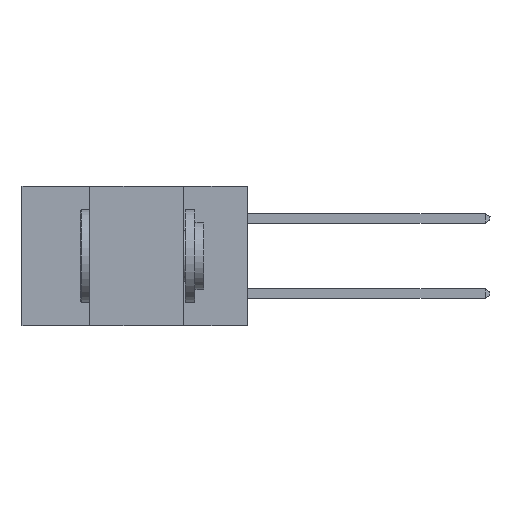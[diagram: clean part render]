
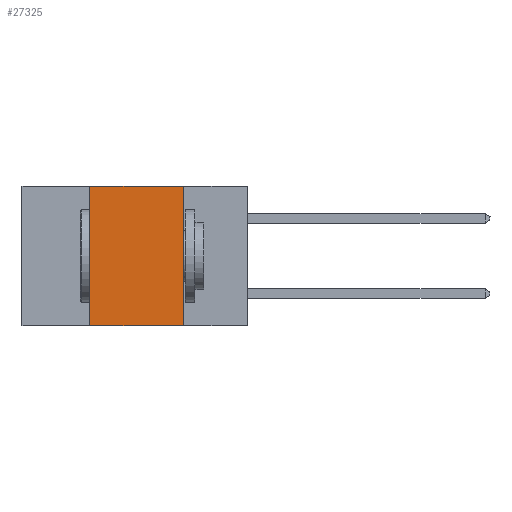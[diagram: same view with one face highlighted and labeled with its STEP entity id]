
A CAD part, left-side view. The second image highlights one B-rep face of the part: STEP entity #27325.
In plain terms, the highlighted planar face has unit normal (-1, 0, 0).
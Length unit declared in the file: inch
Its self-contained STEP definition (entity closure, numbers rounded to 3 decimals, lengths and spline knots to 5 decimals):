
#219 = VERTEX_POINT ( 'NONE', #16009 ) ;
#308 = FACE_OUTER_BOUND ( 'NONE', #2154, .T. ) ;
#2025 = LINE ( 'NONE', #21702, #5653 ) ;
#2154 = EDGE_LOOP ( 'NONE', ( #12642, #14668, #5791, #22028 ) ) ;
#2948 = CARTESIAN_POINT ( 'NONE',  ( 0., 0.42, 0. ) ) ;
#4885 = CARTESIAN_POINT ( 'NONE',  ( 0., 0.6, 0. ) ) ;
#5496 = AXIS2_PLACEMENT_3D ( 'NONE', #6332, #11069, #19581 ) ;
#5653 = VECTOR ( 'NONE', #22550, 39.37008 ) ;
#5791 = ORIENTED_EDGE ( 'NONE', *, *, #9092, .F. ) ;
#6332 = CARTESIAN_POINT ( 'NONE',  ( 0., 0.6, 0. ) ) ;
#7459 = CARTESIAN_POINT ( 'NONE',  ( 0., 0.6, -0.37 ) ) ;
#9027 = DIRECTION ( 'NONE',  ( 0., -1., 0. ) ) ;
#9092 = EDGE_CURVE ( 'NONE', #219, #20656, #26140, .T. ) ;
#10754 = CARTESIAN_POINT ( 'NONE',  ( 0., 0.42, -0.37 ) ) ;
#11069 = DIRECTION ( 'NONE',  ( 1., 0., 0. ) ) ;
#12375 = DIRECTION ( 'NONE',  ( 0., 0., 1. ) ) ;
#12642 = ORIENTED_EDGE ( 'NONE', *, *, #17381, .F. ) ;
#12729 = VERTEX_POINT ( 'NONE', #18388 ) ;
#13207 = VECTOR ( 'NONE', #12375, 39.37008 ) ;
#14668 = ORIENTED_EDGE ( 'NONE', *, *, #26474, .F. ) ;
#14904 = VERTEX_POINT ( 'NONE', #17955 ) ;
#15753 = VECTOR ( 'NONE', #22546, 39.37008 ) ;
#16009 = CARTESIAN_POINT ( 'NONE',  ( 0., 0.42, -0.37 ) ) ;
#16107 = EDGE_CURVE ( 'NONE', #219, #14904, #20418, .T. ) ;
#17381 = EDGE_CURVE ( 'NONE', #12729, #14904, #2025, .T. ) ;
#17849 = VECTOR ( 'NONE', #9027, 39.37008 ) ;
#17955 = CARTESIAN_POINT ( 'NONE',  ( 0., 0.17, -0.37 ) ) ;
#18388 = CARTESIAN_POINT ( 'NONE',  ( 0., 0.17, 0. ) ) ;
#19581 = DIRECTION ( 'NONE',  ( 0., 0., -1. ) ) ;
#20418 = LINE ( 'NONE', #7459, #15753 ) ;
#20656 = VERTEX_POINT ( 'NONE', #2948 ) ;
#21702 = CARTESIAN_POINT ( 'NONE',  ( 0., 0.17, -0.37 ) ) ;
#22028 = ORIENTED_EDGE ( 'NONE', *, *, #16107, .T. ) ;
#22546 = DIRECTION ( 'NONE',  ( 0., -1., 0. ) ) ;
#22550 = DIRECTION ( 'NONE',  ( 0., 0., -1. ) ) ;
#24577 = LINE ( 'NONE', #4885, #17849 ) ;
#26140 = LINE ( 'NONE', #10754, #13207 ) ;
#26474 = EDGE_CURVE ( 'NONE', #20656, #12729, #24577, .T. ) ;
#27325 = ADVANCED_FACE ( 'NONE', ( #308 ), #28327, .F. ) ;
#28327 = PLANE ( 'NONE',  #5496 ) ;
